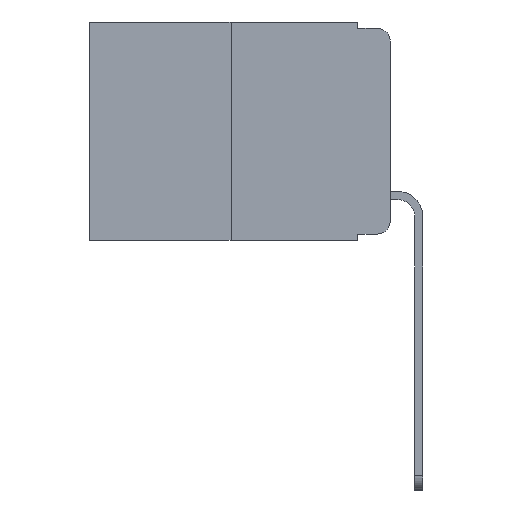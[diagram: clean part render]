
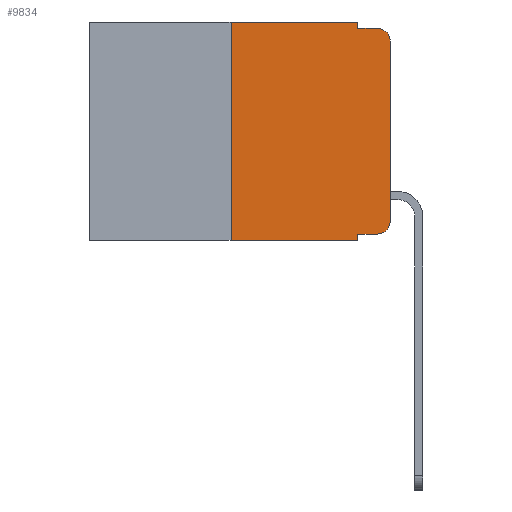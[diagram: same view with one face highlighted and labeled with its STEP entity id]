
A CAD part, left-side view. The second image highlights one B-rep face of the part: STEP entity #9834.
In plain terms, the highlighted planar face has unit normal (-1, 0, 0).
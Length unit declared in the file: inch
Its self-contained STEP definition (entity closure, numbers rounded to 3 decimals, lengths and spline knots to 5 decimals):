
#127 = EDGE_LOOP ( 'NONE', ( #5789, #1070, #8717, #287, #16407, #5333, #6536, #5038, #10291, #5028 ) ) ;
#167 = VERTEX_POINT ( 'NONE', #11483 ) ;
#190 = EDGE_CURVE ( 'NONE', #19536, #9776, #421, .T. ) ;
#287 = ORIENTED_EDGE ( 'NONE', *, *, #1407, .F. ) ;
#369 = VERTEX_POINT ( 'NONE', #4370 ) ;
#421 = LINE ( 'NONE', #6443, #13531 ) ;
#1023 = CARTESIAN_POINT ( 'NONE',  ( 0., 0.473, 0. ) ) ;
#1070 = ORIENTED_EDGE ( 'NONE', *, *, #3696, .T. ) ;
#1407 = EDGE_CURVE ( 'NONE', #10852, #6357, #17948, .T. ) ;
#1692 = DIRECTION ( 'NONE',  ( 0., 0., -1. ) ) ;
#1703 = VECTOR ( 'NONE', #5507, 39.37008 ) ;
#2410 = EDGE_CURVE ( 'NONE', #9776, #10852, #5254, .T. ) ;
#2553 = EDGE_CURVE ( 'NONE', #6357, #14253, #12049, .T. ) ;
#3087 = VECTOR ( 'NONE', #17795, 39.37008 ) ;
#3499 = VERTEX_POINT ( 'NONE', #5327 ) ;
#3589 = CARTESIAN_POINT ( 'NONE',  ( 0., 0.051, 0. ) ) ;
#3696 = EDGE_CURVE ( 'NONE', #369, #14253, #8838, .T. ) ;
#4370 = CARTESIAN_POINT ( 'NONE',  ( 0., 0., -0.03 ) ) ;
#4656 = LINE ( 'NONE', #8531, #3087 ) ;
#4798 = EDGE_CURVE ( 'NONE', #167, #369, #9833, .T. ) ;
#5028 = ORIENTED_EDGE ( 'NONE', *, *, #16737, .T. ) ;
#5038 = ORIENTED_EDGE ( 'NONE', *, *, #18693, .F. ) ;
#5160 = LINE ( 'NONE', #8465, #13105 ) ;
#5254 = LINE ( 'NONE', #1023, #8516 ) ;
#5327 = CARTESIAN_POINT ( 'NONE',  ( 0., 0.051, -0.333 ) ) ;
#5333 = ORIENTED_EDGE ( 'NONE', *, *, #190, .F. ) ;
#5507 = DIRECTION ( 'NONE',  ( 0., 0., -1. ) ) ;
#5605 = VERTEX_POINT ( 'NONE', #14794 ) ;
#5789 = ORIENTED_EDGE ( 'NONE', *, *, #4798, .T. ) ;
#5987 = CIRCLE ( 'NONE', #11596, 0.02 ) ;
#6092 = VERTEX_POINT ( 'NONE', #16740 ) ;
#6267 = CARTESIAN_POINT ( 'NONE',  ( 0., 0., 0. ) ) ;
#6357 = VERTEX_POINT ( 'NONE', #14347 ) ;
#6443 = CARTESIAN_POINT ( 'NONE',  ( 0., 0.25, 0. ) ) ;
#6536 = ORIENTED_EDGE ( 'NONE', *, *, #6560, .T. ) ;
#6560 = EDGE_CURVE ( 'NONE', #19536, #5605, #5160, .T. ) ;
#8465 = CARTESIAN_POINT ( 'NONE',  ( 0., 0.473, -0.343 ) ) ;
#8516 = VECTOR ( 'NONE', #10908, 39.37008 ) ;
#8531 = CARTESIAN_POINT ( 'NONE',  ( 0., 0.051, -0.333 ) ) ;
#8607 = PLANE ( 'NONE',  #9261 ) ;
#8717 = ORIENTED_EDGE ( 'NONE', *, *, #2553, .F. ) ;
#8838 = CIRCLE ( 'NONE', #10157, 0.02 ) ;
#9089 = CARTESIAN_POINT ( 'NONE',  ( 0., 0.051, 0. ) ) ;
#9193 = CARTESIAN_POINT ( 'NONE',  ( 0., 0.02, -0.03 ) ) ;
#9261 = AXIS2_PLACEMENT_3D ( 'NONE', #16310, #19204, #10267 ) ;
#9776 = VERTEX_POINT ( 'NONE', #20396 ) ;
#9834 = ADVANCED_FACE ( 'NONE', ( #15612 ), #8607, .F. ) ;
#9833 = LINE ( 'NONE', #6267, #13433 ) ;
#9876 = VECTOR ( 'NONE', #16746, 39.37008 ) ;
#10157 = AXIS2_PLACEMENT_3D ( 'NONE', #9193, #19795, #10855 ) ;
#10267 = DIRECTION ( 'NONE',  ( 0., 0., -1. ) ) ;
#10291 = ORIENTED_EDGE ( 'NONE', *, *, #17710, .T. ) ;
#10472 = LINE ( 'NONE', #17841, #1703 ) ;
#10852 = VERTEX_POINT ( 'NONE', #3589 ) ;
#10855 = DIRECTION ( 'NONE',  ( 0., 0., -1. ) ) ;
#10908 = DIRECTION ( 'NONE',  ( 0., -1., 0. ) ) ;
#11483 = CARTESIAN_POINT ( 'NONE',  ( 0., 0., -0.313 ) ) ;
#11498 = CARTESIAN_POINT ( 'NONE',  ( 0., 0.051, -0.01 ) ) ;
#11508 = DIRECTION ( 'NONE',  ( -1., 0., 0. ) ) ;
#11596 = AXIS2_PLACEMENT_3D ( 'NONE', #20388, #11508, #1692 ) ;
#11674 = CARTESIAN_POINT ( 'NONE',  ( 0., 0.02, -0.01 ) ) ;
#11716 = DIRECTION ( 'NONE',  ( 0., -1., 0. ) ) ;
#12049 = LINE ( 'NONE', #11498, #19939 ) ;
#12603 = DIRECTION ( 'NONE',  ( 0., 0., 1. ) ) ;
#13105 = VECTOR ( 'NONE', #11716, 39.37008 ) ;
#13433 = VECTOR ( 'NONE', #12603, 39.37008 ) ;
#13531 = VECTOR ( 'NONE', #18276, 39.37008 ) ;
#14253 = VERTEX_POINT ( 'NONE', #11674 ) ;
#14347 = CARTESIAN_POINT ( 'NONE',  ( 0., 0.051, -0.01 ) ) ;
#14456 = DIRECTION ( 'NONE',  ( 0., -1., 0. ) ) ;
#14794 = CARTESIAN_POINT ( 'NONE',  ( 0., 0.051, -0.343 ) ) ;
#15612 = FACE_OUTER_BOUND ( 'NONE', #127, .T. ) ;
#16310 = CARTESIAN_POINT ( 'NONE',  ( 0., 0.473, 0. ) ) ;
#16407 = ORIENTED_EDGE ( 'NONE', *, *, #2410, .F. ) ;
#16737 = EDGE_CURVE ( 'NONE', #6092, #167, #5987, .T. ) ;
#16740 = CARTESIAN_POINT ( 'NONE',  ( 0., 0.02, -0.333 ) ) ;
#16746 = DIRECTION ( 'NONE',  ( 0., 0., -1. ) ) ;
#17710 = EDGE_CURVE ( 'NONE', #3499, #6092, #4656, .T. ) ;
#17795 = DIRECTION ( 'NONE',  ( 0., -1., 0. ) ) ;
#17841 = CARTESIAN_POINT ( 'NONE',  ( 0., 0.051, 0. ) ) ;
#17948 = LINE ( 'NONE', #9089, #9876 ) ;
#18276 = DIRECTION ( 'NONE',  ( 0., 0., 1. ) ) ;
#18693 = EDGE_CURVE ( 'NONE', #3499, #5605, #10472, .T. ) ;
#19204 = DIRECTION ( 'NONE',  ( 1., 0., 0. ) ) ;
#19226 = CARTESIAN_POINT ( 'NONE',  ( 0., 0.25, -0.343 ) ) ;
#19536 = VERTEX_POINT ( 'NONE', #19226 ) ;
#19795 = DIRECTION ( 'NONE',  ( -1., 0., 0. ) ) ;
#19939 = VECTOR ( 'NONE', #14456, 39.37008 ) ;
#20388 = CARTESIAN_POINT ( 'NONE',  ( 0., 0.02, -0.313 ) ) ;
#20396 = CARTESIAN_POINT ( 'NONE',  ( 0., 0.25, 0. ) ) ;
